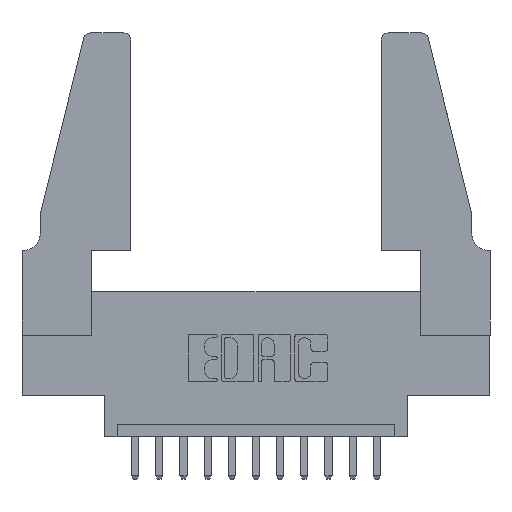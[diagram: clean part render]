
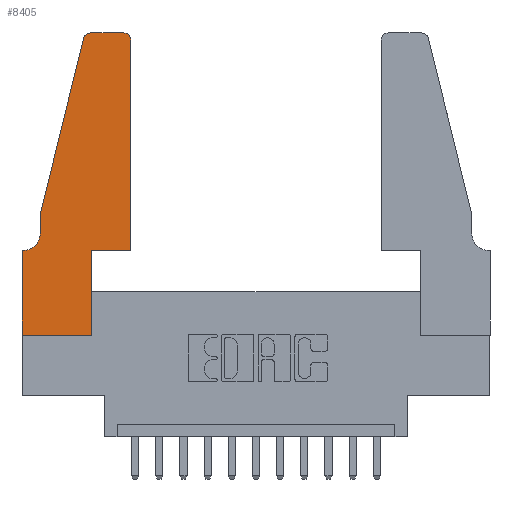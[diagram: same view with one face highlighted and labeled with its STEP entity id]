
A CAD part, top view. The second image highlights one B-rep face of the part: STEP entity #8405.
In plain terms, the highlighted planar face has unit normal (0, 0, 1).
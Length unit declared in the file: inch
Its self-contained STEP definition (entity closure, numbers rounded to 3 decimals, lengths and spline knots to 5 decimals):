
#466 = DIRECTION ( 'NONE',  ( 1., 0., 0. ) ) ;
#772 = CARTESIAN_POINT ( 'NONE',  ( 0.4505, 1.22, 0.37 ) ) ;
#943 = EDGE_CURVE ( 'NONE', #9140, #2252, #10947, .T. ) ;
#1068 = DIRECTION ( 'NONE',  ( 0., 0., -1. ) ) ;
#1107 = VECTOR ( 'NONE', #13358, 39.37008 ) ;
#1172 = LINE ( 'NONE', #11218, #4421 ) ;
#1563 = CIRCLE ( 'NONE', #8920, 0.03 ) ;
#1774 = CARTESIAN_POINT ( 'NONE',  ( 0., 0.35, 0.37 ) ) ;
#1877 = CARTESIAN_POINT ( 'NONE',  ( 0.4505, 0.35, 0.37 ) ) ;
#2172 = CARTESIAN_POINT ( 'NONE',  ( 0., 0., 0.37 ) ) ;
#2191 = CARTESIAN_POINT ( 'NONE',  ( 0.2865, 0.35, 0.37 ) ) ;
#2252 = VERTEX_POINT ( 'NONE', #10965 ) ;
#2311 = DIRECTION ( 'NONE',  ( 0., -1., 0. ) ) ;
#2522 = VECTOR ( 'NONE', #5486, 39.37008 ) ;
#2689 = VERTEX_POINT ( 'NONE', #2172 ) ;
#2728 = EDGE_CURVE ( 'NONE', #6815, #6647, #12141, .T. ) ;
#3177 = EDGE_CURVE ( 'NONE', #9217, #11325, #1172, .T. ) ;
#3382 = VERTEX_POINT ( 'NONE', #13511 ) ;
#3389 = CARTESIAN_POINT ( 'NONE',  ( 0.0755, 0.5, 0.37 ) ) ;
#3390 = EDGE_CURVE ( 'NONE', #11325, #10099, #12480, .T. ) ;
#3456 = DIRECTION ( 'NONE',  ( 0., -1., 0. ) ) ;
#3679 = ORIENTED_EDGE ( 'NONE', *, *, #6211, .T. ) ;
#3817 = EDGE_CURVE ( 'NONE', #2252, #5890, #5844, .T. ) ;
#4130 = ORIENTED_EDGE ( 'NONE', *, *, #943, .T. ) ;
#4362 = DIRECTION ( 'NONE',  ( 1., 0., 0. ) ) ;
#4380 = CARTESIAN_POINT ( 'NONE',  ( 0.0055, 0.42, 0.37 ) ) ;
#4421 = VECTOR ( 'NONE', #4362, 39.37008 ) ;
#4883 = DIRECTION ( 'NONE',  ( 0., 0., 1. ) ) ;
#5310 = CARTESIAN_POINT ( 'NONE',  ( 0., 0., 0.37 ) ) ;
#5486 = DIRECTION ( 'NONE',  ( -1., 0., 0. ) ) ;
#5707 = CARTESIAN_POINT ( 'NONE',  ( 0.0755, 0.5, 0.37 ) ) ;
#5727 = EDGE_LOOP ( 'NONE', ( #12196, #14390, #4130, #7682, #7528, #10581, #10365, #3679, #8801, #6563, #6605, #13759 ) ) ;
#5760 = DIRECTION ( 'NONE',  ( -0.239, -0.971, 0. ) ) ;
#5844 = LINE ( 'NONE', #3389, #9597 ) ;
#5890 = VERTEX_POINT ( 'NONE', #13593 ) ;
#5911 = EDGE_CURVE ( 'NONE', #8613, #8736, #11690, .T. ) ;
#6004 = CARTESIAN_POINT ( 'NONE',  ( 0.284, 1.25, 0.37 ) ) ;
#6211 = EDGE_CURVE ( 'NONE', #2689, #3382, #13671, .T. ) ;
#6563 = ORIENTED_EDGE ( 'NONE', *, *, #3177, .T. ) ;
#6574 = DIRECTION ( 'NONE',  ( 0., 1., 0. ) ) ;
#6605 = ORIENTED_EDGE ( 'NONE', *, *, #3390, .T. ) ;
#6647 = VERTEX_POINT ( 'NONE', #6004 ) ;
#6815 = VERTEX_POINT ( 'NONE', #13523 ) ;
#6836 = VECTOR ( 'NONE', #7072, 39.37008 ) ;
#7072 = DIRECTION ( 'NONE',  ( 0., 1., 0. ) ) ;
#7265 = AXIS2_PLACEMENT_3D ( 'NONE', #9716, #8821, #13470 ) ;
#7308 = VECTOR ( 'NONE', #12444, 39.37008 ) ;
#7528 = ORIENTED_EDGE ( 'NONE', *, *, #7970, .T. ) ;
#7682 = ORIENTED_EDGE ( 'NONE', *, *, #3817, .T. ) ;
#7970 = EDGE_CURVE ( 'NONE', #5890, #8613, #13539, .T. ) ;
#8405 = ADVANCED_FACE ( 'NONE', ( #10830 ), #13048, .T. ) ;
#8549 = DIRECTION ( 'NONE',  ( 1., 0., 0. ) ) ;
#8613 = VERTEX_POINT ( 'NONE', #10203 ) ;
#8736 = VERTEX_POINT ( 'NONE', #14267 ) ;
#8744 = AXIS2_PLACEMENT_3D ( 'NONE', #1774, #12118, #8549 ) ;
#8801 = ORIENTED_EDGE ( 'NONE', *, *, #11194, .T. ) ;
#8821 = DIRECTION ( 'NONE',  ( 0., 0., 1. ) ) ;
#8920 = AXIS2_PLACEMENT_3D ( 'NONE', #11761, #4883, #466 ) ;
#9140 = VERTEX_POINT ( 'NONE', #11337 ) ;
#9160 = VECTOR ( 'NONE', #5760, 39.37008 ) ;
#9217 = VERTEX_POINT ( 'NONE', #14725 ) ;
#9258 = VECTOR ( 'NONE', #6574, 39.37008 ) ;
#9409 = CARTESIAN_POINT ( 'NONE',  ( 0.4505, 0.35, 0.37 ) ) ;
#9597 = VECTOR ( 'NONE', #2311, 39.37008 ) ;
#9716 = CARTESIAN_POINT ( 'NONE',  ( 0.284, 1.22, 0.37 ) ) ;
#9796 = EDGE_CURVE ( 'NONE', #6647, #9140, #12908, .T. ) ;
#10099 = VERTEX_POINT ( 'NONE', #772 ) ;
#10203 = CARTESIAN_POINT ( 'NONE',  ( 0.0055, 0.35, 0.37 ) ) ;
#10365 = ORIENTED_EDGE ( 'NONE', *, *, #12055, .T. ) ;
#10411 = LINE ( 'NONE', #2191, #6836 ) ;
#10581 = ORIENTED_EDGE ( 'NONE', *, *, #5911, .T. ) ;
#10830 = FACE_OUTER_BOUND ( 'NONE', #5727, .T. ) ;
#10947 = LINE ( 'NONE', #5707, #9160 ) ;
#10965 = CARTESIAN_POINT ( 'NONE',  ( 0.0755, 0.5, 0.37 ) ) ;
#11194 = EDGE_CURVE ( 'NONE', #3382, #9217, #10411, .T. ) ;
#11218 = CARTESIAN_POINT ( 'NONE',  ( 0.4505, 0.35, 0.37 ) ) ;
#11325 = VERTEX_POINT ( 'NONE', #9409 ) ;
#11337 = CARTESIAN_POINT ( 'NONE',  ( 0.25487, 1.22718, 0.37 ) ) ;
#11462 = VECTOR ( 'NONE', #3456, 39.37008 ) ;
#11690 = LINE ( 'NONE', #13635, #2522 ) ;
#11736 = AXIS2_PLACEMENT_3D ( 'NONE', #4380, #1068, #13741 ) ;
#11761 = CARTESIAN_POINT ( 'NONE',  ( 0.4205, 1.22, 0.37 ) ) ;
#12055 = EDGE_CURVE ( 'NONE', #8736, #2689, #14499, .T. ) ;
#12118 = DIRECTION ( 'NONE',  ( 0., 0., 1. ) ) ;
#12141 = LINE ( 'NONE', #12302, #7308 ) ;
#12196 = ORIENTED_EDGE ( 'NONE', *, *, #2728, .T. ) ;
#12302 = CARTESIAN_POINT ( 'NONE',  ( 0.2605, 1.25, 0.37 ) ) ;
#12444 = DIRECTION ( 'NONE',  ( -1., 0., 0. ) ) ;
#12480 = LINE ( 'NONE', #1877, #9258 ) ;
#12908 = CIRCLE ( 'NONE', #7265, 0.03 ) ;
#13048 = PLANE ( 'NONE',  #8744 ) ;
#13358 = DIRECTION ( 'NONE',  ( 1., 0., 0. ) ) ;
#13470 = DIRECTION ( 'NONE',  ( 1., 0., 0. ) ) ;
#13502 = EDGE_CURVE ( 'NONE', #10099, #6815, #1563, .T. ) ;
#13511 = CARTESIAN_POINT ( 'NONE',  ( 0.2865, 0., 0.37 ) ) ;
#13523 = CARTESIAN_POINT ( 'NONE',  ( 0.4205, 1.25, 0.37 ) ) ;
#13539 = CIRCLE ( 'NONE', #11736, 0.07 ) ;
#13593 = CARTESIAN_POINT ( 'NONE',  ( 0.0755, 0.42, 0.37 ) ) ;
#13635 = CARTESIAN_POINT ( 'NONE',  ( 0.0755, 0.35, 0.37 ) ) ;
#13671 = LINE ( 'NONE', #5310, #1107 ) ;
#13741 = DIRECTION ( 'NONE',  ( -1., 0., 0. ) ) ;
#13759 = ORIENTED_EDGE ( 'NONE', *, *, #13502, .T. ) ;
#14064 = CARTESIAN_POINT ( 'NONE',  ( 0., 0., 0.37 ) ) ;
#14267 = CARTESIAN_POINT ( 'NONE',  ( 0., 0.35, 0.37 ) ) ;
#14390 = ORIENTED_EDGE ( 'NONE', *, *, #9796, .T. ) ;
#14499 = LINE ( 'NONE', #14064, #11462 ) ;
#14725 = CARTESIAN_POINT ( 'NONE',  ( 0.2865, 0.35, 0.37 ) ) ;
